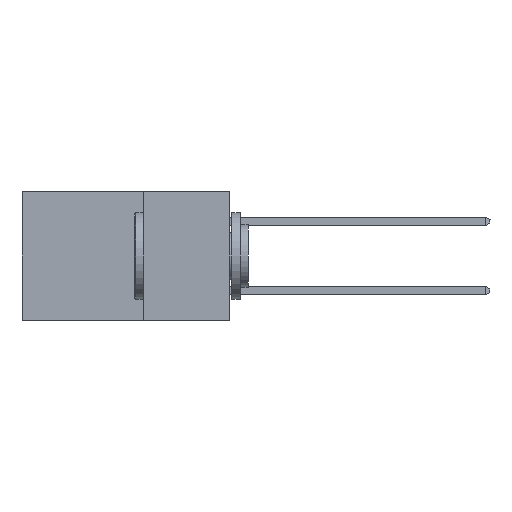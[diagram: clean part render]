
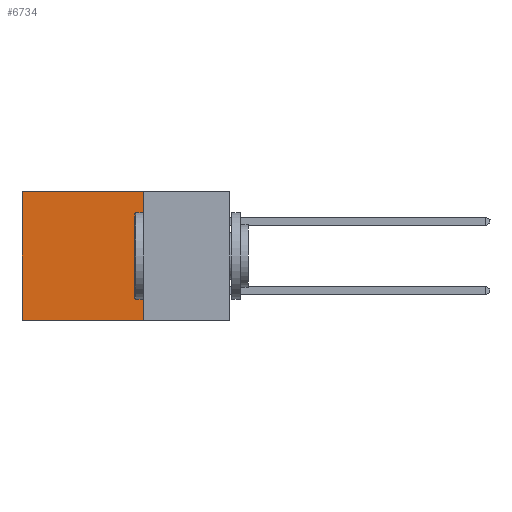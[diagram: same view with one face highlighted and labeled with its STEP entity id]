
A CAD part, left-side view. The second image highlights one B-rep face of the part: STEP entity #6734.
In plain terms, the highlighted planar face has unit normal (-1, 0, 0).
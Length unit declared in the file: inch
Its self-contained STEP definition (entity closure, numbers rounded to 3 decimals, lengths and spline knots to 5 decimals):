
#1483 = LINE ( 'NONE', #4617, #20742 ) ;
#1652 = ORIENTED_EDGE ( 'NONE', *, *, #13064, .T. ) ;
#1835 = EDGE_CURVE ( 'NONE', #32066, #27270, #26875, .T. ) ;
#3420 = LINE ( 'NONE', #12852, #13244 ) ;
#3624 = ORIENTED_EDGE ( 'NONE', *, *, #12929, .F. ) ;
#3933 = LINE ( 'NONE', #25995, #11787 ) ;
#4617 = CARTESIAN_POINT ( 'NONE',  ( 0.298, 0.25, 0. ) ) ;
#5563 = VERTEX_POINT ( 'NONE', #5588 ) ;
#5588 = CARTESIAN_POINT ( 'NONE',  ( 0.298, 0.6, 0. ) ) ;
#5861 = EDGE_LOOP ( 'NONE', ( #23680, #28956, #3624, #1652 ) ) ;
#6734 = ADVANCED_FACE ( 'NONE', ( #18308 ), #12976, .F. ) ;
#6957 = DIRECTION ( 'NONE',  ( 0., 1., 0. ) ) ;
#7160 = DIRECTION ( 'NONE',  ( 0., 0., -1. ) ) ;
#7929 = CARTESIAN_POINT ( 'NONE',  ( 0.298, 0.25, 0. ) ) ;
#8750 = CARTESIAN_POINT ( 'NONE',  ( 0.298, 0.25, -0.37 ) ) ;
#10412 = CARTESIAN_POINT ( 'NONE',  ( 0.298, 0.25, 0. ) ) ;
#11787 = VECTOR ( 'NONE', #13673, 39.37008 ) ;
#12852 = CARTESIAN_POINT ( 'NONE',  ( 0.298, 0.25, 0. ) ) ;
#12929 = EDGE_CURVE ( 'NONE', #22862, #32066, #1483, .T. ) ;
#12976 = PLANE ( 'NONE',  #27236 ) ;
#13064 = EDGE_CURVE ( 'NONE', #22862, #5563, #3420, .T. ) ;
#13244 = VECTOR ( 'NONE', #27784, 39.37008 ) ;
#13673 = DIRECTION ( 'NONE',  ( 0., 0., -1. ) ) ;
#18308 = FACE_OUTER_BOUND ( 'NONE', #5861, .T. ) ;
#18345 = DIRECTION ( 'NONE',  ( 0., 0., -1. ) ) ;
#20190 = VECTOR ( 'NONE', #6957, 39.37008 ) ;
#20742 = VECTOR ( 'NONE', #7160, 39.37008 ) ;
#22862 = VERTEX_POINT ( 'NONE', #10412 ) ;
#23077 = EDGE_CURVE ( 'NONE', #5563, #27270, #3933, .T. ) ;
#23680 = ORIENTED_EDGE ( 'NONE', *, *, #23077, .T. ) ;
#25707 = DIRECTION ( 'NONE',  ( 1., 0., 0. ) ) ;
#25995 = CARTESIAN_POINT ( 'NONE',  ( 0.298, 0.6, 0. ) ) ;
#26739 = CARTESIAN_POINT ( 'NONE',  ( 0.298, 0.25, -0.37 ) ) ;
#26875 = LINE ( 'NONE', #8750, #20190 ) ;
#27236 = AXIS2_PLACEMENT_3D ( 'NONE', #7929, #25707, #18345 ) ;
#27270 = VERTEX_POINT ( 'NONE', #31206 ) ;
#27784 = DIRECTION ( 'NONE',  ( 0., 1., 0. ) ) ;
#28956 = ORIENTED_EDGE ( 'NONE', *, *, #1835, .F. ) ;
#31206 = CARTESIAN_POINT ( 'NONE',  ( 0.298, 0.6, -0.37 ) ) ;
#32066 = VERTEX_POINT ( 'NONE', #26739 ) ;
